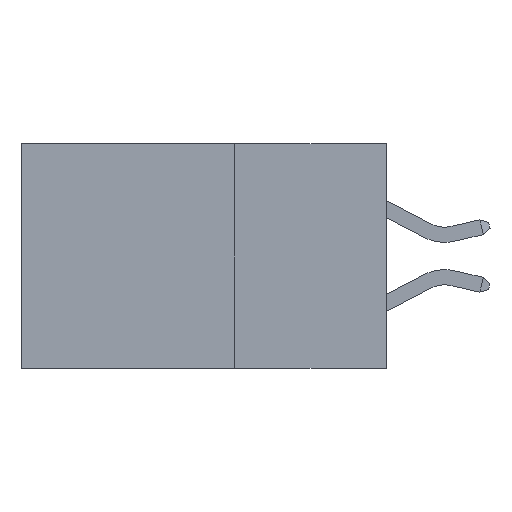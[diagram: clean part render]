
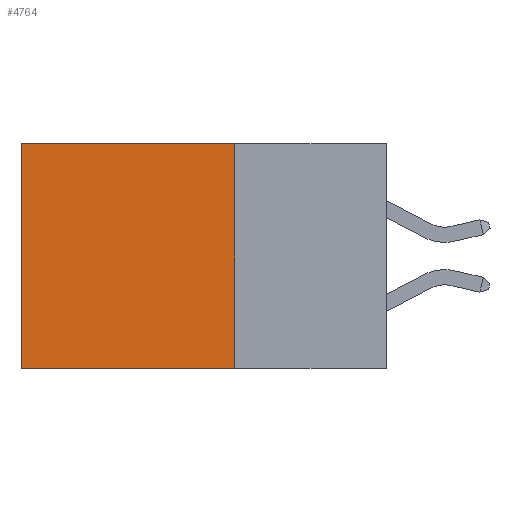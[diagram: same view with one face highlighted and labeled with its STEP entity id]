
A CAD part, left-side view. The second image highlights one B-rep face of the part: STEP entity #4764.
In plain terms, the highlighted planar face has unit normal (-1, 0, 0).
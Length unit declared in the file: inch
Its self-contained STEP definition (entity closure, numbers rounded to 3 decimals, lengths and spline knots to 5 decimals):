
#378 = LINE ( 'NONE', #16711, #5778 ) ;
#713 = VERTEX_POINT ( 'NONE', #6651 ) ;
#1041 = EDGE_LOOP ( 'NONE', ( #6800, #16092, #17488, #16070 ) ) ;
#1589 = FACE_OUTER_BOUND ( 'NONE', #1041, .T. ) ;
#1802 = CARTESIAN_POINT ( 'NONE',  ( 0.2615, 0.25, 0. ) ) ;
#2096 = CARTESIAN_POINT ( 'NONE',  ( 0.2615, 0.6, -0.37 ) ) ;
#3066 = VERTEX_POINT ( 'NONE', #2096 ) ;
#3463 = DIRECTION ( 'NONE',  ( 0., 0., -1. ) ) ;
#3526 = EDGE_CURVE ( 'NONE', #6634, #3066, #13280, .T. ) ;
#4165 = DIRECTION ( 'NONE',  ( 0., 1., 0. ) ) ;
#4290 = DIRECTION ( 'NONE',  ( 0., 0., -1. ) ) ;
#4764 = ADVANCED_FACE ( 'NONE', ( #1589 ), #7390, .F. ) ;
#4790 = VECTOR ( 'NONE', #3463, 39.37008 ) ;
#4855 = CARTESIAN_POINT ( 'NONE',  ( 0.2615, 0.25, -0.37 ) ) ;
#5011 = CARTESIAN_POINT ( 'NONE',  ( 0.2615, 0.25, -0.37 ) ) ;
#5204 = LINE ( 'NONE', #14671, #4790 ) ;
#5778 = VECTOR ( 'NONE', #4290, 39.37008 ) ;
#5945 = DIRECTION ( 'NONE',  ( 1., 0., 0. ) ) ;
#6634 = VERTEX_POINT ( 'NONE', #4855 ) ;
#6651 = CARTESIAN_POINT ( 'NONE',  ( 0.2615, 0.6, 0. ) ) ;
#6800 = ORIENTED_EDGE ( 'NONE', *, *, #12311, .T. ) ;
#7390 = PLANE ( 'NONE',  #9900 ) ;
#8397 = CARTESIAN_POINT ( 'NONE',  ( 0.2615, 0.25, -0.37 ) ) ;
#8517 = VERTEX_POINT ( 'NONE', #1802 ) ;
#9878 = DIRECTION ( 'NONE',  ( 0., 0., -1. ) ) ;
#9900 = AXIS2_PLACEMENT_3D ( 'NONE', #8397, #5945, #9878 ) ;
#12311 = EDGE_CURVE ( 'NONE', #713, #3066, #5204, .T. ) ;
#13134 = VECTOR ( 'NONE', #4165, 39.37008 ) ;
#13280 = LINE ( 'NONE', #5011, #15914 ) ;
#13722 = LINE ( 'NONE', #16667, #13134 ) ;
#14653 = EDGE_CURVE ( 'NONE', #8517, #6634, #378, .T. ) ;
#14671 = CARTESIAN_POINT ( 'NONE',  ( 0.2615, 0.6, -0.37 ) ) ;
#15914 = VECTOR ( 'NONE', #17693, 39.37008 ) ;
#16070 = ORIENTED_EDGE ( 'NONE', *, *, #18008, .T. ) ;
#16092 = ORIENTED_EDGE ( 'NONE', *, *, #3526, .F. ) ;
#16667 = CARTESIAN_POINT ( 'NONE',  ( 0.2615, 0.25, 0. ) ) ;
#16711 = CARTESIAN_POINT ( 'NONE',  ( 0.2615, 0.25, -0.37 ) ) ;
#17488 = ORIENTED_EDGE ( 'NONE', *, *, #14653, .F. ) ;
#17693 = DIRECTION ( 'NONE',  ( 0., 1., 0. ) ) ;
#18008 = EDGE_CURVE ( 'NONE', #8517, #713, #13722, .T. ) ;
